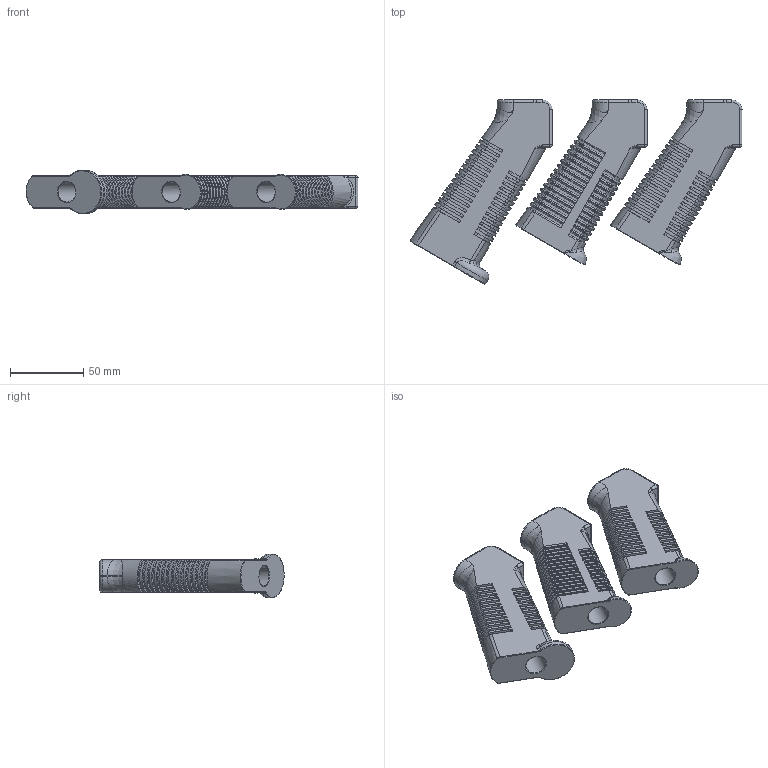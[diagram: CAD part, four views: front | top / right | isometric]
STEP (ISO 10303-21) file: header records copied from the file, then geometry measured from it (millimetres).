
FILE_DESCRIPTION(/* description */ (''),/* implementation_level */ '2;1');
FILE_NAME(/* name */ 'GRIP X.stp',/* time_stamp */ '2020-10-02T16:49:39+03:00',/* author */ (''),/* organization */ (''),/* preprocessor_version */ 'ST-DEVELOPER v15.2',/* originating_system */ 'Autodesk Translator Framework v2.0.0.5431',/* authorisation */ '');
FILE_SCHEMA (('AUTOMOTIVE_DESIGN { 1 0 10303 214 3 1 1 }'));
Products named in the file (1): GRIP X4
Bounding box: 227.33 x 126.14 x 30.06 mm (x, y, z)
Volume: 253095.1 mm3; surface area: 72882.9 mm2
Topology: 3 solids, 3 shells, 1347 faces, 3726 edges, 2379 vertices
Faces by surface type: bspline 723, plane 379, cylinder 220, torus 13, cone 6, sphere 6
Full cylindrical faces by diameter (mm): 3.8 x3, 6 x2, 6.5 x1, 14 x3
Entity records: 81196 total; most frequent: CARTESIAN_POINT 52604, ORIENTED_EDGE 7404, EDGE_CURVE 3702, DIRECTION 3674, VERTEX_POINT 2373, B_SPLINE_CURVE_WITH_KNOTS 2002, EDGE_LOOP 1365, AXIS2_PLACEMENT_3D 1349
